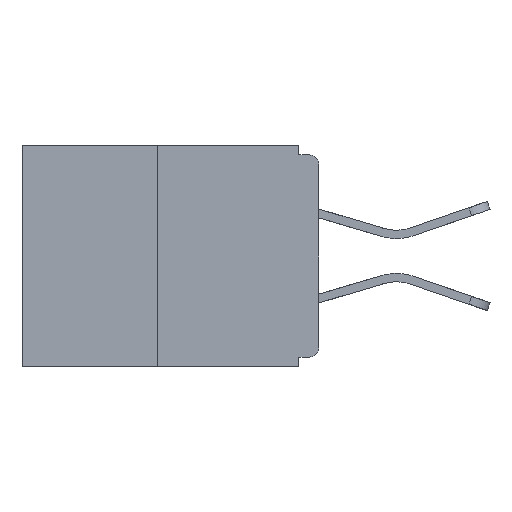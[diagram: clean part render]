
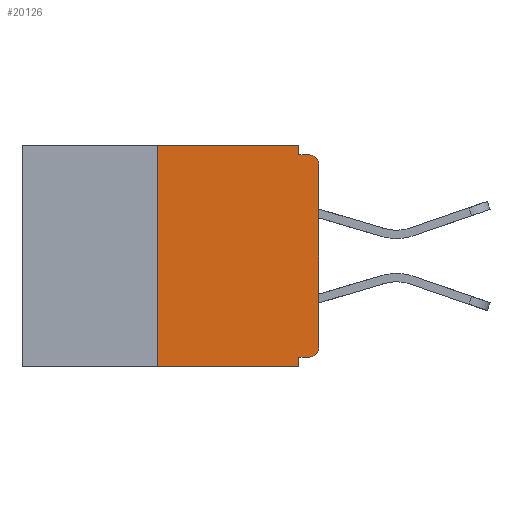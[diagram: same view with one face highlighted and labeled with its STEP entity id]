
A CAD part, left-side view. The second image highlights one B-rep face of the part: STEP entity #20126.
In plain terms, the highlighted planar face has unit normal (-1, 0, 0).
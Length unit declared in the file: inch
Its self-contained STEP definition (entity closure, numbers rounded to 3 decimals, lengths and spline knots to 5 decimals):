
#95 = LINE ( 'NONE', #13187, #8690 ) ;
#855 = DIRECTION ( 'NONE',  ( 0., 0., -1. ) ) ;
#1232 = VERTEX_POINT ( 'NONE', #19541 ) ;
#1402 = EDGE_CURVE ( 'NONE', #10424, #9054, #7706, .T. ) ;
#1800 = DIRECTION ( 'NONE',  ( 0., 0., -1. ) ) ;
#2458 = CARTESIAN_POINT ( 'NONE',  ( 0., 0.015, -0.313 ) ) ;
#2537 = ORIENTED_EDGE ( 'NONE', *, *, #9629, .F. ) ;
#2968 = LINE ( 'NONE', #16167, #11143 ) ;
#3602 = VERTEX_POINT ( 'NONE', #8149 ) ;
#3668 = LINE ( 'NONE', #6731, #8557 ) ;
#3752 = VERTEX_POINT ( 'NONE', #15553 ) ;
#4300 = DIRECTION ( 'NONE',  ( -1., 0., 0. ) ) ;
#4637 = EDGE_LOOP ( 'NONE', ( #15228, #18494, #5051, #2537, #8452, #6349, #14250, #11908, #20754, #12314 ) ) ;
#5051 = ORIENTED_EDGE ( 'NONE', *, *, #8864, .T. ) ;
#5589 = EDGE_CURVE ( 'NONE', #3752, #18581, #5820, .T. ) ;
#5749 = EDGE_CURVE ( 'NONE', #17271, #18866, #2968, .T. ) ;
#5820 = LINE ( 'NONE', #17277, #20857 ) ;
#6349 = ORIENTED_EDGE ( 'NONE', *, *, #1402, .T. ) ;
#6731 = CARTESIAN_POINT ( 'NONE',  ( 0., 0., 0. ) ) ;
#7706 = CIRCLE ( 'NONE', #16050, 0.015 ) ;
#8080 = DIRECTION ( 'NONE',  ( 1., 0., 0. ) ) ;
#8135 = DIRECTION ( 'NONE',  ( -1., 0., 0. ) ) ;
#8149 = CARTESIAN_POINT ( 'NONE',  ( 0., 0.031, -0.328 ) ) ;
#8452 = ORIENTED_EDGE ( 'NONE', *, *, #9129, .F. ) ;
#8557 = VECTOR ( 'NONE', #20008, 39.37008 ) ;
#8690 = VECTOR ( 'NONE', #10258, 39.37008 ) ;
#8864 = EDGE_CURVE ( 'NONE', #17271, #13272, #95, .T. ) ;
#8880 = DIRECTION ( 'NONE',  ( 0., -1., 0. ) ) ;
#9054 = VERTEX_POINT ( 'NONE', #18725 ) ;
#9129 = EDGE_CURVE ( 'NONE', #10424, #3602, #9470, .T. ) ;
#9470 = LINE ( 'NONE', #21008, #14653 ) ;
#9629 = EDGE_CURVE ( 'NONE', #3602, #13272, #19306, .T. ) ;
#9800 = VECTOR ( 'NONE', #21480, 39.37008 ) ;
#10158 = DIRECTION ( 'NONE',  ( 0., 0., -1. ) ) ;
#10258 = DIRECTION ( 'NONE',  ( 0., -1., 0. ) ) ;
#10424 = VERTEX_POINT ( 'NONE', #21088 ) ;
#10909 = CARTESIAN_POINT ( 'NONE',  ( 0., 0.015, -0.015 ) ) ;
#10999 = EDGE_CURVE ( 'NONE', #18866, #17424, #16480, .T. ) ;
#11054 = CARTESIAN_POINT ( 'NONE',  ( 0., 0.031, -0.343 ) ) ;
#11143 = VECTOR ( 'NONE', #19320, 39.37008 ) ;
#11348 = FACE_OUTER_BOUND ( 'NONE', #4637, .T. ) ;
#11526 = CARTESIAN_POINT ( 'NONE',  ( 0., 0.015, -0.03 ) ) ;
#11695 = CARTESIAN_POINT ( 'NONE',  ( 0., 0.46, 0. ) ) ;
#11908 = ORIENTED_EDGE ( 'NONE', *, *, #15445, .T. ) ;
#12070 = VECTOR ( 'NONE', #855, 39.37008 ) ;
#12314 = ORIENTED_EDGE ( 'NONE', *, *, #13502, .F. ) ;
#12404 = AXIS2_PLACEMENT_3D ( 'NONE', #11526, #8135, #1800 ) ;
#12471 = EDGE_CURVE ( 'NONE', #9054, #1232, #3668, .T. ) ;
#12586 = CARTESIAN_POINT ( 'NONE',  ( 0., 0.031, -0.343 ) ) ;
#13187 = CARTESIAN_POINT ( 'NONE',  ( 0., 0.46, -0.343 ) ) ;
#13272 = VERTEX_POINT ( 'NONE', #11054 ) ;
#13439 = CIRCLE ( 'NONE', #12404, 0.015 ) ;
#13502 = EDGE_CURVE ( 'NONE', #17424, #3752, #21234, .T. ) ;
#14250 = ORIENTED_EDGE ( 'NONE', *, *, #12471, .T. ) ;
#14653 = VECTOR ( 'NONE', #17736, 39.37008 ) ;
#15228 = ORIENTED_EDGE ( 'NONE', *, *, #10999, .F. ) ;
#15445 = EDGE_CURVE ( 'NONE', #1232, #18581, #13439, .T. ) ;
#15553 = CARTESIAN_POINT ( 'NONE',  ( 0., 0.031, -0.015 ) ) ;
#15904 = CARTESIAN_POINT ( 'NONE',  ( 0., 0.031, 0. ) ) ;
#16050 = AXIS2_PLACEMENT_3D ( 'NONE', #2458, #4300, #20988 ) ;
#16167 = CARTESIAN_POINT ( 'NONE',  ( 0., 0.25, 0. ) ) ;
#16480 = LINE ( 'NONE', #11695, #9800 ) ;
#16609 = AXIS2_PLACEMENT_3D ( 'NONE', #19829, #8080, #10158 ) ;
#17271 = VERTEX_POINT ( 'NONE', #18892 ) ;
#17277 = CARTESIAN_POINT ( 'NONE',  ( 0., 0., -0.015 ) ) ;
#17424 = VERTEX_POINT ( 'NONE', #17478 ) ;
#17453 = VECTOR ( 'NONE', #19424, 39.37008 ) ;
#17478 = CARTESIAN_POINT ( 'NONE',  ( 0., 0.031, 0. ) ) ;
#17736 = DIRECTION ( 'NONE',  ( 0., 1., 0. ) ) ;
#18494 = ORIENTED_EDGE ( 'NONE', *, *, #5749, .F. ) ;
#18581 = VERTEX_POINT ( 'NONE', #10909 ) ;
#18725 = CARTESIAN_POINT ( 'NONE',  ( 0., 0., -0.313 ) ) ;
#18866 = VERTEX_POINT ( 'NONE', #20124 ) ;
#18892 = CARTESIAN_POINT ( 'NONE',  ( 0., 0.25, -0.343 ) ) ;
#19306 = LINE ( 'NONE', #12586, #17453 ) ;
#19320 = DIRECTION ( 'NONE',  ( 0., 0., 1. ) ) ;
#19424 = DIRECTION ( 'NONE',  ( 0., 0., -1. ) ) ;
#19541 = CARTESIAN_POINT ( 'NONE',  ( 0., 0., -0.03 ) ) ;
#19829 = CARTESIAN_POINT ( 'NONE',  ( 0., 0.46, 0. ) ) ;
#20008 = DIRECTION ( 'NONE',  ( 0., 0., 1. ) ) ;
#20124 = CARTESIAN_POINT ( 'NONE',  ( 0., 0.25, 0. ) ) ;
#20126 = ADVANCED_FACE ( 'NONE', ( #11348 ), #21456, .F. ) ;
#20754 = ORIENTED_EDGE ( 'NONE', *, *, #5589, .F. ) ;
#20857 = VECTOR ( 'NONE', #8880, 39.37008 ) ;
#20988 = DIRECTION ( 'NONE',  ( 0., 0., -1. ) ) ;
#21008 = CARTESIAN_POINT ( 'NONE',  ( 0., 0., -0.328 ) ) ;
#21088 = CARTESIAN_POINT ( 'NONE',  ( 0., 0.015, -0.328 ) ) ;
#21234 = LINE ( 'NONE', #15904, #12070 ) ;
#21456 = PLANE ( 'NONE',  #16609 ) ;
#21480 = DIRECTION ( 'NONE',  ( 0., -1., 0. ) ) ;
